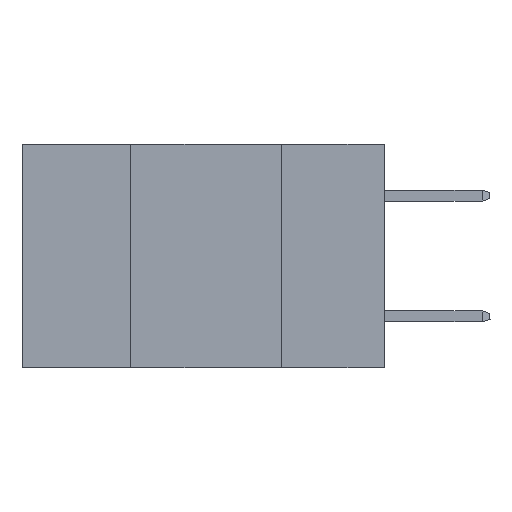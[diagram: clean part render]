
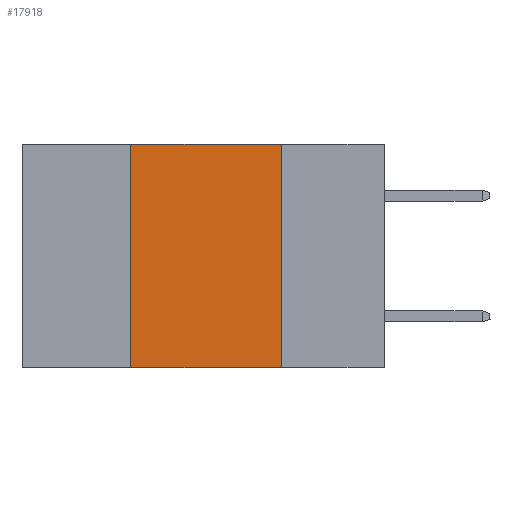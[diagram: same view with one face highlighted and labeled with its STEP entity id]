
A CAD part, left-side view. The second image highlights one B-rep face of the part: STEP entity #17918.
In plain terms, the highlighted planar face has unit normal (-1, 0, 0).
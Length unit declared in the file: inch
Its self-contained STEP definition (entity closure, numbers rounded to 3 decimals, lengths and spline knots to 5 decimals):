
#651 = VERTEX_POINT ( 'NONE', #7304 ) ;
#1296 = EDGE_LOOP ( 'NONE', ( #3786, #6185, #11842, #4921 ) ) ;
#1938 = CARTESIAN_POINT ( 'NONE',  ( 0., 0.6, 0. ) ) ;
#3193 = VECTOR ( 'NONE', #14387, 39.37008 ) ;
#3374 = CARTESIAN_POINT ( 'NONE',  ( 0., 0.42, -0.37 ) ) ;
#3641 = DIRECTION ( 'NONE',  ( 1., 0., 0. ) ) ;
#3697 = CARTESIAN_POINT ( 'NONE',  ( 0., 0.6, -0.37 ) ) ;
#3786 = ORIENTED_EDGE ( 'NONE', *, *, #9100, .F. ) ;
#4885 = DIRECTION ( 'NONE',  ( 0., -1., 0. ) ) ;
#4921 = ORIENTED_EDGE ( 'NONE', *, *, #11862, .T. ) ;
#6185 = ORIENTED_EDGE ( 'NONE', *, *, #19718, .F. ) ;
#6954 = CARTESIAN_POINT ( 'NONE',  ( 0., 0.42, 0. ) ) ;
#7304 = CARTESIAN_POINT ( 'NONE',  ( 0., 0.17, 0. ) ) ;
#7481 = LINE ( 'NONE', #9602, #11600 ) ;
#9100 = EDGE_CURVE ( 'NONE', #651, #18066, #7481, .T. ) ;
#9393 = LINE ( 'NONE', #14220, #10372 ) ;
#9602 = CARTESIAN_POINT ( 'NONE',  ( 0., 0.17, -0.37 ) ) ;
#10285 = CARTESIAN_POINT ( 'NONE',  ( 0., 0.17, -0.37 ) ) ;
#10372 = VECTOR ( 'NONE', #4885, 39.37008 ) ;
#11139 = LINE ( 'NONE', #3374, #3193 ) ;
#11170 = DIRECTION ( 'NONE',  ( 0., 0., -1. ) ) ;
#11504 = PLANE ( 'NONE',  #20218 ) ;
#11556 = DIRECTION ( 'NONE',  ( 0., -1., 0. ) ) ;
#11600 = VECTOR ( 'NONE', #11170, 39.37008 ) ;
#11842 = ORIENTED_EDGE ( 'NONE', *, *, #19083, .F. ) ;
#11862 = EDGE_CURVE ( 'NONE', #15207, #18066, #15464, .T. ) ;
#14220 = CARTESIAN_POINT ( 'NONE',  ( 0., 0.6, 0. ) ) ;
#14387 = DIRECTION ( 'NONE',  ( 0., 0., 1. ) ) ;
#14652 = DIRECTION ( 'NONE',  ( 0., 0., -1. ) ) ;
#14955 = VECTOR ( 'NONE', #11556, 39.37008 ) ;
#15207 = VERTEX_POINT ( 'NONE', #17514 ) ;
#15464 = LINE ( 'NONE', #3697, #14955 ) ;
#16118 = VERTEX_POINT ( 'NONE', #6954 ) ;
#17514 = CARTESIAN_POINT ( 'NONE',  ( 0., 0.42, -0.37 ) ) ;
#17918 = ADVANCED_FACE ( 'NONE', ( #20394 ), #11504, .F. ) ;
#18066 = VERTEX_POINT ( 'NONE', #10285 ) ;
#19083 = EDGE_CURVE ( 'NONE', #15207, #16118, #11139, .T. ) ;
#19718 = EDGE_CURVE ( 'NONE', #16118, #651, #9393, .T. ) ;
#20218 = AXIS2_PLACEMENT_3D ( 'NONE', #1938, #3641, #14652 ) ;
#20394 = FACE_OUTER_BOUND ( 'NONE', #1296, .T. ) ;
